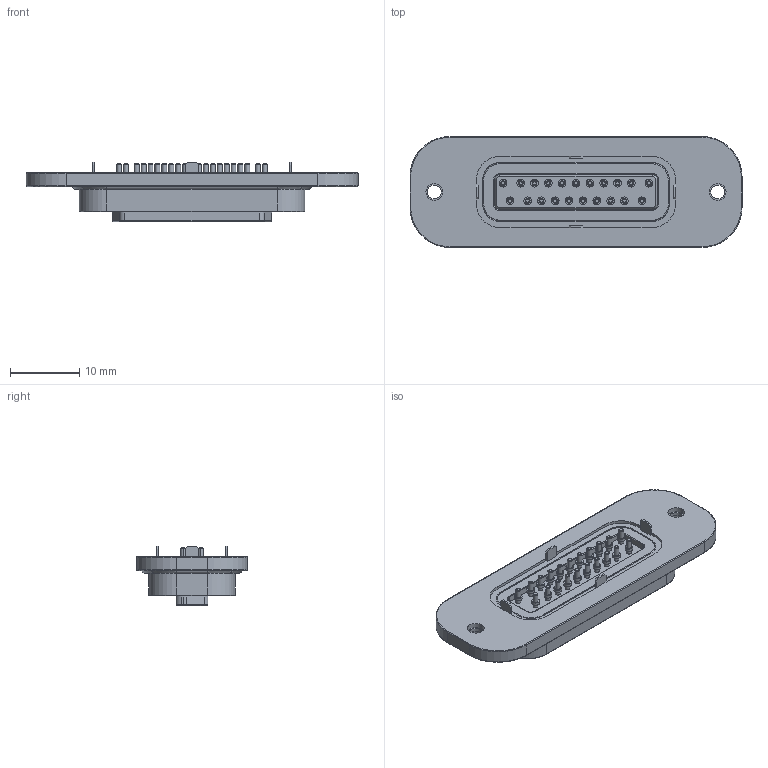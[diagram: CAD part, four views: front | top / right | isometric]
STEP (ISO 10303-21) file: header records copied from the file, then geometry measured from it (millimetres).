
FILE_DESCRIPTION (( 'STEP AP214' ), '1' );
FILE_NAME ('686A2131260114E.STEP', '2023-04-26T14:40:32', ( '' ), ( '' ), 'SwSTEP 2.0', 'SolidWorks 2020', '' );
FILE_SCHEMA (( 'AUTOMOTIVE_DESIGN' ));
Length unit declared in the file: millimetre
Products named in the file (1): 686A2131260114E
Bounding box: 48 x 16.04 x 8.55 mm (x, y, z)
Volume: 2869.6 mm3; surface area: 3948 mm2
Topology: 2 solids, 2 shells, 683 faces, 1550 edges, 944 vertices
Faces by surface type: cylinder 319, plane 197, cone 117, bspline 50
Entity records: 21793 total; most frequent: CARTESIAN_POINT 4202, DIRECTION 3511, ORIENTED_EDGE 2974, EDGE_CURVE 1487, AXIS2_PLACEMENT_3D 1433, VERTEX_POINT 944, EDGE_LOOP 825, CIRCLE 799
